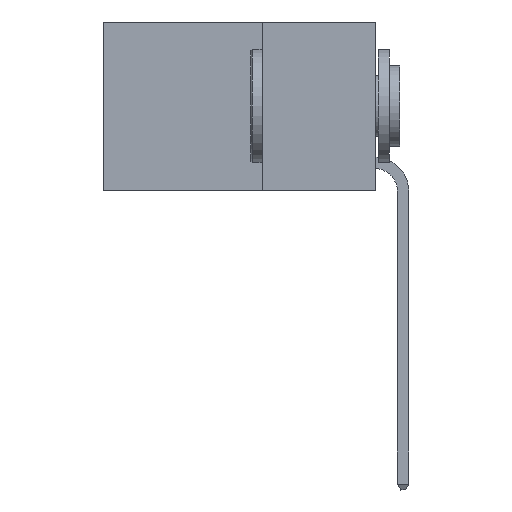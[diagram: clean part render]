
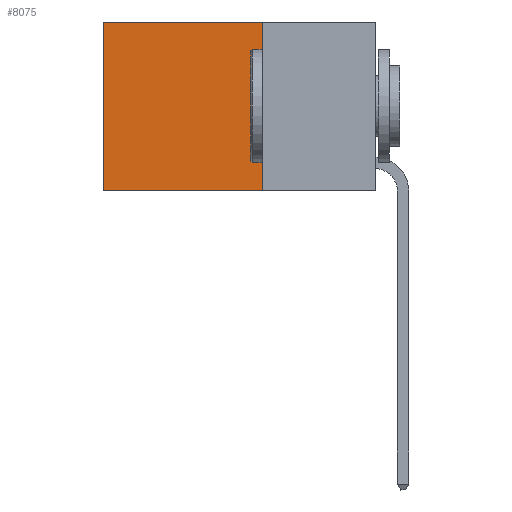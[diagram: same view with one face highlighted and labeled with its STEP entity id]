
A CAD part, left-side view. The second image highlights one B-rep face of the part: STEP entity #8075.
In plain terms, the highlighted planar face has unit normal (-1, 0, 0).
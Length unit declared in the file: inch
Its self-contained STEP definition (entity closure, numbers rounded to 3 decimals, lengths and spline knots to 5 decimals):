
#48 = EDGE_CURVE ( 'NONE', #6738, #650, #7841, .T. ) ;
#215 = CARTESIAN_POINT ( 'NONE',  ( 0.2625, 0.25, -0.37 ) ) ;
#650 = VERTEX_POINT ( 'NONE', #5321 ) ;
#964 = CARTESIAN_POINT ( 'NONE',  ( 0.2625, 0.25, 0. ) ) ;
#1055 = EDGE_CURVE ( 'NONE', #6738, #3971, #14347, .T. ) ;
#2063 = VECTOR ( 'NONE', #12580, 39.37008 ) ;
#3103 = PLANE ( 'NONE',  #13257 ) ;
#3430 = EDGE_LOOP ( 'NONE', ( #13333, #4797, #9666, #11395 ) ) ;
#3971 = VERTEX_POINT ( 'NONE', #6485 ) ;
#4449 = VECTOR ( 'NONE', #15019, 39.37008 ) ;
#4797 = ORIENTED_EDGE ( 'NONE', *, *, #9147, .F. ) ;
#5254 = CARTESIAN_POINT ( 'NONE',  ( 0.2625, 0.25, 0. ) ) ;
#5321 = CARTESIAN_POINT ( 'NONE',  ( 0.2625, 0.25, -0.37 ) ) ;
#5481 = DIRECTION ( 'NONE',  ( 0., 0., -1. ) ) ;
#5520 = VECTOR ( 'NONE', #11911, 39.37008 ) ;
#6485 = CARTESIAN_POINT ( 'NONE',  ( 0.2625, 0.6, 0. ) ) ;
#6612 = CARTESIAN_POINT ( 'NONE',  ( 0.2625, 0.25, 0. ) ) ;
#6738 = VERTEX_POINT ( 'NONE', #5254 ) ;
#6964 = EDGE_CURVE ( 'NONE', #3971, #14875, #13640, .T. ) ;
#7096 = DIRECTION ( 'NONE',  ( 0., 1., 0. ) ) ;
#7841 = LINE ( 'NONE', #964, #4449 ) ;
#8075 = ADVANCED_FACE ( 'NONE', ( #13549 ), #3103, .F. ) ;
#8377 = LINE ( 'NONE', #215, #9509 ) ;
#9147 = EDGE_CURVE ( 'NONE', #650, #14875, #8377, .T. ) ;
#9215 = CARTESIAN_POINT ( 'NONE',  ( 0.2625, 0.6, 0. ) ) ;
#9509 = VECTOR ( 'NONE', #7096, 39.37008 ) ;
#9666 = ORIENTED_EDGE ( 'NONE', *, *, #48, .F. ) ;
#10926 = CARTESIAN_POINT ( 'NONE',  ( 0.2625, 0.25, 0. ) ) ;
#11276 = DIRECTION ( 'NONE',  ( 1., 0., 0. ) ) ;
#11395 = ORIENTED_EDGE ( 'NONE', *, *, #1055, .T. ) ;
#11911 = DIRECTION ( 'NONE',  ( 0., 1., 0. ) ) ;
#12580 = DIRECTION ( 'NONE',  ( 0., 0., -1. ) ) ;
#13257 = AXIS2_PLACEMENT_3D ( 'NONE', #6612, #11276, #5481 ) ;
#13333 = ORIENTED_EDGE ( 'NONE', *, *, #6964, .T. ) ;
#13549 = FACE_OUTER_BOUND ( 'NONE', #3430, .T. ) ;
#13640 = LINE ( 'NONE', #9215, #2063 ) ;
#14347 = LINE ( 'NONE', #10926, #5520 ) ;
#14720 = CARTESIAN_POINT ( 'NONE',  ( 0.2625, 0.6, -0.37 ) ) ;
#14875 = VERTEX_POINT ( 'NONE', #14720 ) ;
#15019 = DIRECTION ( 'NONE',  ( 0., 0., -1. ) ) ;
